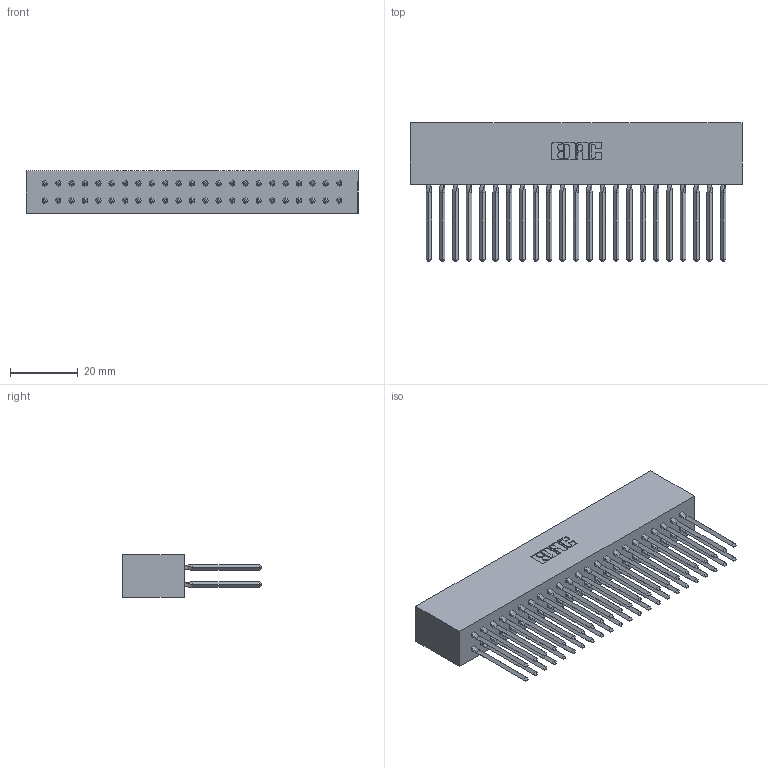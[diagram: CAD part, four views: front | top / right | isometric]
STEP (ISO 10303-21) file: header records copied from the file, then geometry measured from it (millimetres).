
FILE_DESCRIPTION (( 'STEP AP203' ), '1' );
FILE_NAME ('317-046-543-801.STEP', '2020-02-28T02:32:17', ( '' ), ( '' ), 'SwSTEP 2.0', 'SolidWorks 2016', '' );
FILE_SCHEMA (( 'CONFIG_CONTROL_DESIGN' ));
Length unit declared in the file: inch
Products named in the file (3): 317 Part_Lugless; 317-046-543-801; 317-290-001_543
Assembly tree (47 placements, depth 2):
  317-046-543-801
    317 Part_Lugless
    317-290-001_543  x46
Bounding box: 98.35 x 41.15 x 12.7 mm (x, y, z)
Volume: 17886.1 mm3; surface area: 26665.5 mm2
Topology: 47 solids, 47 shells, 4184 faces, 11601 edges, 7472 vertices
Faces by surface type: plane 3408, cylinder 592, bspline 184
Entity records: 35488 total; most frequent: CARTESIAN_POINT 6603, ORIENTED_EDGE 6102, DIRECTION 5085, EDGE_CURVE 3051, LINE 2803, VECTOR 2803, VERTEX_POINT 2027, AXIS2_PLACEMENT_3D 1141
